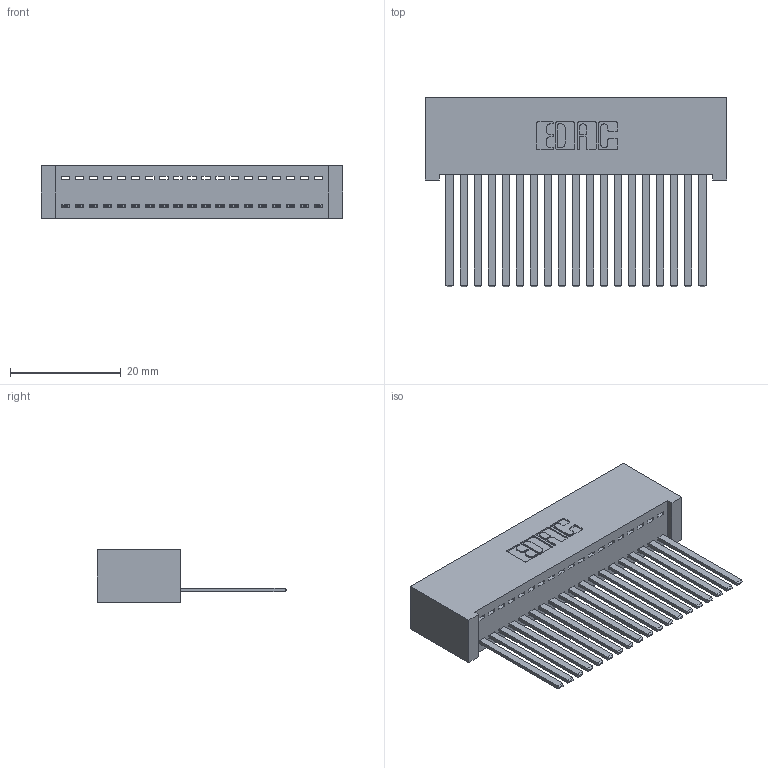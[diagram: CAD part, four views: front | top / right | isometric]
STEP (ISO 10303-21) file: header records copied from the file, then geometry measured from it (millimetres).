
FILE_DESCRIPTION (( 'STEP AP203' ), '1' );
FILE_NAME ('342-019-544-101.STEP', '2019-10-01T20:40:01', ( '' ), ( '' ), 'SwSTEP 2.0', 'SolidWorks 2016', '' );
FILE_SCHEMA (( 'CONFIG_CONTROL_DESIGN' ));
Length unit declared in the file: inch
Products named in the file (3): 342 Part_Lugless; 345-292-001_345-293-144; 342-019-544-101
Assembly tree (20 placements, depth 2):
  342-019-544-101
    342 Part_Lugless
    345-292-001_345-293-144  x19
Bounding box: 54.51 x 34.3 x 9.4 mm (x, y, z)
Volume: 5323.6 mm3; surface area: 8337.6 mm2
Topology: 20 solids, 20 shells, 1090 faces, 3277 edges, 2158 vertices
Faces by surface type: plane 784, cylinder 306
Entity records: 13997 total; most frequent: CARTESIAN_POINT 2423, ORIENTED_EDGE 2378, DIRECTION 2079, EDGE_CURVE 1189, LINE 1073, VECTOR 1073, VERTEX_POINT 790, AXIS2_PLACEMENT_3D 503
